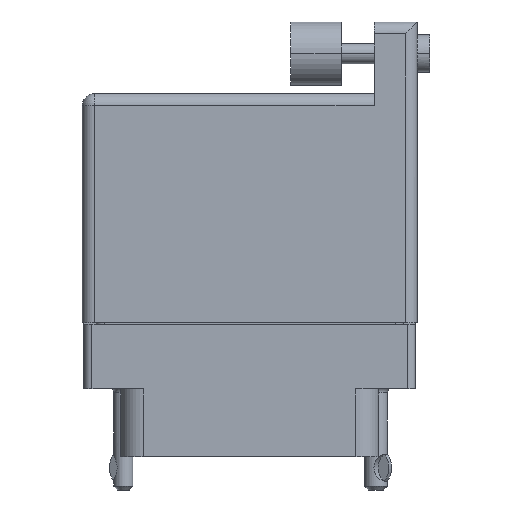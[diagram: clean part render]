
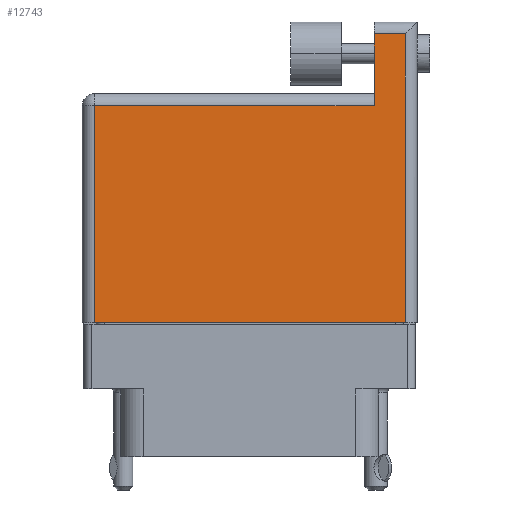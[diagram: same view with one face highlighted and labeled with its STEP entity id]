
A CAD part, front view. The second image highlights one B-rep face of the part: STEP entity #12743.
In plain terms, the highlighted face is planar.
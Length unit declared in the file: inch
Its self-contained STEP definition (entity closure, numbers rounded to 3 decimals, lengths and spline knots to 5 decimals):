
#47 = ORIENTED_EDGE ( 'NONE', *, *, #5221, .T. ) ;
#197 = DIRECTION ( 'NONE',  ( 0., 1., 0. ) ) ;
#1946 = ORIENTED_EDGE ( 'NONE', *, *, #14117, .T. ) ;
#2384 = VECTOR ( 'NONE', #18123, 39.37008 ) ;
#3491 = CARTESIAN_POINT ( 'NONE',  ( -0.6625, 0.806, 0.3575 ) ) ;
#5221 = EDGE_CURVE ( 'NONE', #11712, #21618, #20123, .T. ) ;
#5392 = DIRECTION ( 'NONE',  ( 1., 0., 0. ) ) ;
#5447 = CARTESIAN_POINT ( 'NONE',  ( -0.6155, -0.1, 0.3575 ) ) ;
#5750 = DIRECTION ( 'NONE',  ( -1., 0., 0. ) ) ;
#5846 = VERTEX_POINT ( 'NONE', #30461 ) ;
#5910 = VECTOR ( 'NONE', #197, 39.37008 ) ;
#5982 = DIRECTION ( 'NONE',  ( -1., 0., 0. ) ) ;
#6316 = PLANE ( 'NONE',  #12810 ) ;
#6519 = VECTOR ( 'NONE', #13150, 39.37008 ) ;
#6808 = EDGE_CURVE ( 'NONE', #26849, #35319, #33324, .T. ) ;
#7080 = CARTESIAN_POINT ( 'NONE',  ( 0.4925, 1.09, 0.3575 ) ) ;
#7897 = ORIENTED_EDGE ( 'NONE', *, *, #14566, .T. ) ;
#8611 = CARTESIAN_POINT ( 'NONE',  ( -0.6625, 0.759, 0.3575 ) ) ;
#8629 = VERTEX_POINT ( 'NONE', #31524 ) ;
#9609 = CARTESIAN_POINT ( 'NONE',  ( 0.6155, -0.1, 0.3575 ) ) ;
#9647 = EDGE_LOOP ( 'NONE', ( #47, #7897, #19173, #1946, #35588, #11817 ) ) ;
#9930 = CARTESIAN_POINT ( 'NONE',  ( 0.6155, 1.043, 0.3575 ) ) ;
#11712 = VERTEX_POINT ( 'NONE', #37422 ) ;
#11817 = ORIENTED_EDGE ( 'NONE', *, *, #20924, .T. ) ;
#12743 = ADVANCED_FACE ( 'NONE', ( #21632 ), #6316, .F. ) ;
#12810 = AXIS2_PLACEMENT_3D ( 'NONE', #3491, #31475, #31678 ) ;
#13150 = DIRECTION ( 'NONE',  ( 0., -1., 0. ) ) ;
#14117 = EDGE_CURVE ( 'NONE', #35319, #5846, #19168, .T. ) ;
#14566 = EDGE_CURVE ( 'NONE', #21618, #26849, #18523, .T. ) ;
#18123 = DIRECTION ( 'NONE',  ( 0., -1., 0. ) ) ;
#18523 = LINE ( 'NONE', #18930, #5910 ) ;
#18627 = CARTESIAN_POINT ( 'NONE',  ( 0.4925, 1.043, 0.3575 ) ) ;
#18930 = CARTESIAN_POINT ( 'NONE',  ( 0.6155, 1.09, 0.3575 ) ) ;
#19168 = LINE ( 'NONE', #7080, #6519 ) ;
#19173 = ORIENTED_EDGE ( 'NONE', *, *, #6808, .T. ) ;
#20123 = LINE ( 'NONE', #23720, #28951 ) ;
#20924 = EDGE_CURVE ( 'NONE', #8629, #11712, #27573, .T. ) ;
#21292 = LINE ( 'NONE', #8611, #30023 ) ;
#21618 = VERTEX_POINT ( 'NONE', #9609 ) ;
#21632 = FACE_OUTER_BOUND ( 'NONE', #9647, .T. ) ;
#23720 = CARTESIAN_POINT ( 'NONE',  ( -0.6625, -0.1, 0.3575 ) ) ;
#24825 = CARTESIAN_POINT ( 'NONE',  ( 0.4925, 1.043, 0.3575 ) ) ;
#26849 = VERTEX_POINT ( 'NONE', #9930 ) ;
#27573 = LINE ( 'NONE', #5447, #2384 ) ;
#28951 = VECTOR ( 'NONE', #5392, 39.37008 ) ;
#29128 = EDGE_CURVE ( 'NONE', #5846, #8629, #21292, .T. ) ;
#30023 = VECTOR ( 'NONE', #5982, 39.37008 ) ;
#30461 = CARTESIAN_POINT ( 'NONE',  ( 0.4925, 0.759, 0.3575 ) ) ;
#31475 = DIRECTION ( 'NONE',  ( 0., 0., -1. ) ) ;
#31524 = CARTESIAN_POINT ( 'NONE',  ( -0.6155, 0.759, 0.3575 ) ) ;
#31678 = DIRECTION ( 'NONE',  ( -1., 0., 0. ) ) ;
#33324 = LINE ( 'NONE', #18627, #38522 ) ;
#35319 = VERTEX_POINT ( 'NONE', #24825 ) ;
#35588 = ORIENTED_EDGE ( 'NONE', *, *, #29128, .T. ) ;
#37422 = CARTESIAN_POINT ( 'NONE',  ( -0.6155, -0.1, 0.3575 ) ) ;
#38522 = VECTOR ( 'NONE', #5750, 39.37008 ) ;
